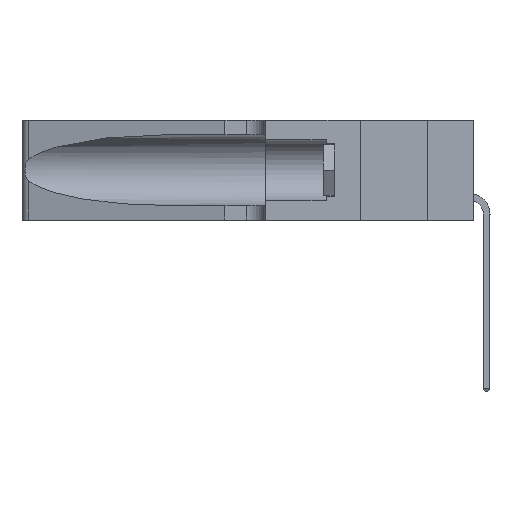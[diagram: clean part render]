
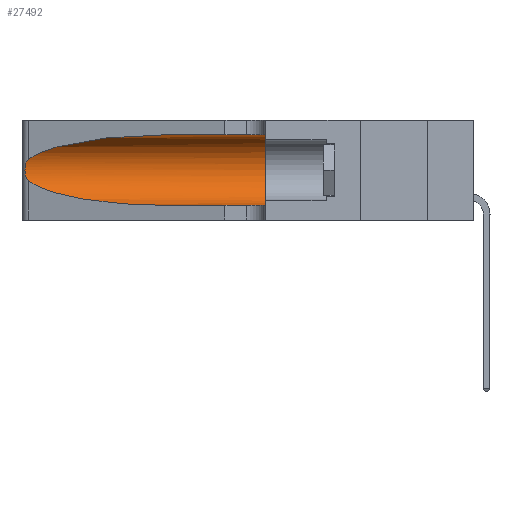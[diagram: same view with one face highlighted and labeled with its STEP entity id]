
A CAD part, left-side view. The second image highlights one B-rep face of the part: STEP entity #27492.
In plain terms, the highlighted cylindrical face has radius 3.308 mm (diameter 6.617 mm), a partial arc.
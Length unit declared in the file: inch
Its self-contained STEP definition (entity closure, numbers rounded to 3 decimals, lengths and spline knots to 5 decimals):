
#275 = EDGE_CURVE ( 'NONE', #3785, #44316, #6049, .T. ) ;
#828 = CARTESIAN_POINT ( 'NONE',  ( 0.2373, 1.15595, 0.28018 ) ) ;
#1152 = CARTESIAN_POINT ( 'NONE',  ( 0.25487, 1.22718, 0.22369 ) ) ;
#1553 = DIRECTION ( 'NONE',  ( 0., -1., 0. ) ) ;
#2483 = DIRECTION ( 'NONE',  ( 0., 0., 1. ) ) ;
#2730 = CARTESIAN_POINT ( 'NONE',  ( 0.25856, 1.23593, 0.16098 ) ) ;
#2944 = CARTESIAN_POINT ( 'NONE',  ( 0.1305, 0.35, 0.05475 ) ) ;
#3049 = CARTESIAN_POINT ( 'NONE',  ( 0.25854, 1.2359, 0.20912 ) ) ;
#3673 = CIRCLE ( 'NONE', #23101, 0.13025 ) ;
#3686 =( BOUNDED_CURVE ( )  B_SPLINE_CURVE ( 3, ( #22626, #15104, #828, #1152 ),
 .UNSPECIFIED., .F., .F. ) 
 B_SPLINE_CURVE_WITH_KNOTS ( ( 4, 4 ),
 ( 1.5708, 2.84003 ),
 .UNSPECIFIED. ) 
 CURVE ( )  GEOMETRIC_REPRESENTATION_ITEM ( )  RATIONAL_B_SPLINE_CURVE ( ( 1., 0.87, 0.87, 1. ) ) 
 REPRESENTATION_ITEM ( '' )  );
#3785 = VERTEX_POINT ( 'NONE', #13059 ) ;
#5685 = ORIENTED_EDGE ( 'NONE', *, *, #24782, .T. ) ;
#6018 = CARTESIAN_POINT ( 'NONE',  ( 0.26018, 1.23835, 0.19895 ) ) ;
#6049 = LINE ( 'NONE', #45641, #26170 ) ;
#6549 = EDGE_CURVE ( 'NONE', #40349, #3785, #34397, .T. ) ;
#6636 = DIRECTION ( 'NONE',  ( 0., -1., 0. ) ) ;
#10104 = CARTESIAN_POINT ( 'NONE',  ( 0.25639, 1.23184, 0.21858 ) ) ;
#10815 = VERTEX_POINT ( 'NONE', #17587 ) ;
#13059 = CARTESIAN_POINT ( 'NONE',  ( 0.1305, 0.72297, 0.05475 ) ) ;
#13728 = CARTESIAN_POINT ( 'NONE',  ( 0.25789, 1.23486, 0.15765 ) ) ;
#15104 = CARTESIAN_POINT ( 'NONE',  ( 0.18966, 0.96281, 0.31525 ) ) ;
#16416 = DIRECTION ( 'NONE',  ( 0., 1., 0. ) ) ;
#16565 = CARTESIAN_POINT ( 'NONE',  ( 0.1305, 0.35, 0.31525 ) ) ;
#16812 = DIRECTION ( 'NONE',  ( 0., 0., -1. ) ) ;
#17297 = CARTESIAN_POINT ( 'NONE',  ( 0.25555, 1.22993, 0.14849 ) ) ;
#17587 = CARTESIAN_POINT ( 'NONE',  ( 0.25487, 1.22718, 0.22369 ) ) ;
#17788 = CARTESIAN_POINT ( 'NONE',  ( 0.2373, 1.15595, 0.08982 ) ) ;
#19188 = LINE ( 'NONE', #44477, #41661 ) ;
#20444 = CARTESIAN_POINT ( 'NONE',  ( 0.25487, 1.22718, 0.22369 ) ) ;
#20753 = ORIENTED_EDGE ( 'NONE', *, *, #41400, .F. ) ;
#20903 = CARTESIAN_POINT ( 'NONE',  ( 0.25487, 1.22718, 0.14631 ) ) ;
#20927 = CARTESIAN_POINT ( 'NONE',  ( 0.25487, 1.22718, 0.14631 ) ) ;
#21085 = CARTESIAN_POINT ( 'NONE',  ( 0.18966, 0.96281, 0.05475 ) ) ;
#22382 = CARTESIAN_POINT ( 'NONE',  ( 0.25487, 1.22718, 0.14631 ) ) ;
#22442 = ORIENTED_EDGE ( 'NONE', *, *, #42649, .T. ) ;
#22626 = CARTESIAN_POINT ( 'NONE',  ( 0.1305, 0.72297, 0.31525 ) ) ;
#23101 = AXIS2_PLACEMENT_3D ( 'NONE', #41337, #16416, #2483 ) ;
#24027 = CARTESIAN_POINT ( 'NONE',  ( 0.1305, 1.61858, 0.185 ) ) ;
#24195 = CARTESIAN_POINT ( 'NONE',  ( 0.26075, 1.23896, 0.178 ) ) ;
#24241 = CYLINDRICAL_SURFACE ( 'NONE', #34536, 0.13025 ) ;
#24674 = CARTESIAN_POINT ( 'NONE',  ( 0.1305, 0.72297, 0.05475 ) ) ;
#24782 = EDGE_CURVE ( 'NONE', #41060, #10815, #3686, .T. ) ;
#26170 = VECTOR ( 'NONE', #6636, 39.37008 ) ;
#27492 = ADVANCED_FACE ( 'NONE', ( #31500 ), #24241, .F. ) ;
#27779 = CARTESIAN_POINT ( 'NONE',  ( 0.25787, 1.23484, 0.2124 ) ) ;
#28306 = EDGE_CURVE ( 'NONE', #30642, #44316, #3673, .T. ) ;
#30642 = VERTEX_POINT ( 'NONE', #16565 ) ;
#31263 = EDGE_LOOP ( 'NONE', ( #5685, #22442, #36105, #40974, #42897, #20753 ) ) ;
#31500 = FACE_OUTER_BOUND ( 'NONE', #31263, .T. ) ;
#34397 =( BOUNDED_CURVE ( )  B_SPLINE_CURVE ( 3, ( #20927, #17788, #21085, #24674 ),
 .UNSPECIFIED., .F., .F. ) 
 B_SPLINE_CURVE_WITH_KNOTS ( ( 4, 4 ),
 ( 3.44316, 4.71239 ),
 .UNSPECIFIED. ) 
 CURVE ( )  GEOMETRIC_REPRESENTATION_ITEM ( )  RATIONAL_B_SPLINE_CURVE ( ( 1., 0.87, 0.87, 1. ) ) 
 REPRESENTATION_ITEM ( '' )  );
#34536 = AXIS2_PLACEMENT_3D ( 'NONE', #24027, #41750, #16812 ) ;
#35008 = CARTESIAN_POINT ( 'NONE',  ( 0.26017, 1.23833, 0.17102 ) ) ;
#35156 = CARTESIAN_POINT ( 'NONE',  ( 0.25555, 1.22994, 0.2215 ) ) ;
#36036 = CARTESIAN_POINT ( 'NONE',  ( 0.1305, 0.72297, 0.31525 ) ) ;
#36105 = ORIENTED_EDGE ( 'NONE', *, *, #6549, .T. ) ;
#40349 = VERTEX_POINT ( 'NONE', #22382 ) ;
#40974 = ORIENTED_EDGE ( 'NONE', *, *, #275, .T. ) ;
#41060 = VERTEX_POINT ( 'NONE', #36036 ) ;
#41337 = CARTESIAN_POINT ( 'NONE',  ( 0.1305, 0.35, 0.185 ) ) ;
#41400 = EDGE_CURVE ( 'NONE', #41060, #30642, #19188, .T. ) ;
#41661 = VECTOR ( 'NONE', #1553, 39.37008 ) ;
#41750 = DIRECTION ( 'NONE',  ( 0., -1., 0. ) ) ;
#41899 = B_SPLINE_CURVE_WITH_KNOTS ( 'NONE', 3,
 ( #20444, #35156, #10104, #27779, #3049, #6018, #45492, #24195, #35008, #2730, #13728, #45786, #17297, #20903 ),
 .UNSPECIFIED., .F., .F.,
 ( 4, 2, 2, 2, 2, 2, 4 ),
 ( 0., 0.00027, 0.00053, 0.00107, 0.0016, 0.00187, 0.00214 ),
 .UNSPECIFIED. ) ;
#42649 = EDGE_CURVE ( 'NONE', #10815, #40349, #41899, .T. ) ;
#42897 = ORIENTED_EDGE ( 'NONE', *, *, #28306, .F. ) ;
#44316 = VERTEX_POINT ( 'NONE', #2944 ) ;
#44477 = CARTESIAN_POINT ( 'NONE',  ( 0.1305, 1.61858, 0.31525 ) ) ;
#45492 = CARTESIAN_POINT ( 'NONE',  ( 0.26075, 1.23896, 0.19203 ) ) ;
#45641 = CARTESIAN_POINT ( 'NONE',  ( 0.1305, 1.61858, 0.05475 ) ) ;
#45786 = CARTESIAN_POINT ( 'NONE',  ( 0.25639, 1.23186, 0.15144 ) ) ;
